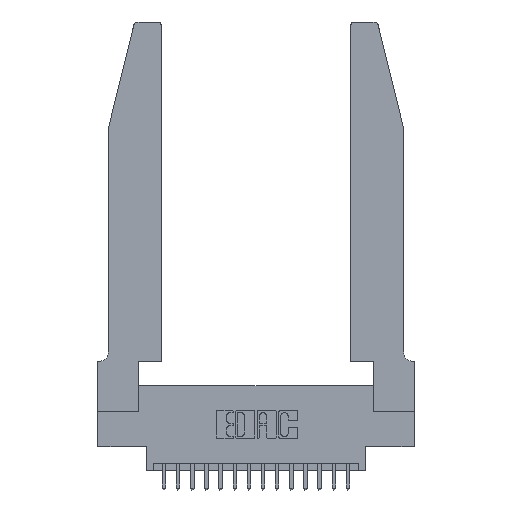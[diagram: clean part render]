
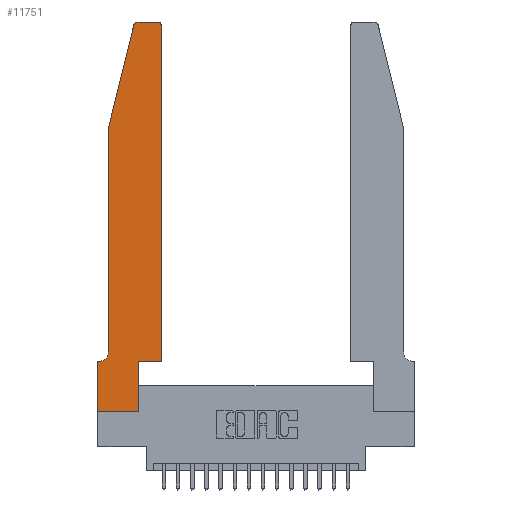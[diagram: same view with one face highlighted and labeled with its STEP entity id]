
A CAD part, top view. The second image highlights one B-rep face of the part: STEP entity #11751.
In plain terms, the highlighted planar face has unit normal (0, 0, 1).
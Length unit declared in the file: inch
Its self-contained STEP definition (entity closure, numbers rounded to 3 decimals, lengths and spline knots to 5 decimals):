
#253 = EDGE_CURVE ( 'NONE', #4071, #18024, #14234, .T. ) ;
#289 = ORIENTED_EDGE ( 'NONE', *, *, #15749, .T. ) ;
#462 = LINE ( 'NONE', #18966, #4676 ) ;
#570 = DIRECTION ( 'NONE',  ( -1., 0., 0. ) ) ;
#686 = CARTESIAN_POINT ( 'NONE',  ( 0.4205, 2.72, 0.37 ) ) ;
#854 = DIRECTION ( 'NONE',  ( 0., 1., 0. ) ) ;
#1380 = VECTOR ( 'NONE', #854, 39.37008 ) ;
#1409 = VERTEX_POINT ( 'NONE', #7134 ) ;
#2099 = DIRECTION ( 'NONE',  ( 1., 0., 0. ) ) ;
#2106 = CARTESIAN_POINT ( 'NONE',  ( 0.4505, 2.72, 0.37 ) ) ;
#2364 = EDGE_CURVE ( 'NONE', #1409, #4262, #3921, .T. ) ;
#2713 = DIRECTION ( 'NONE',  ( 0., 0., 1. ) ) ;
#3007 = CARTESIAN_POINT ( 'NONE',  ( 0.0755, 0.42, 0.37 ) ) ;
#3080 = AXIS2_PLACEMENT_3D ( 'NONE', #18809, #3494, #2099 ) ;
#3386 = CARTESIAN_POINT ( 'NONE',  ( 0.4505, 0.35, 0.37 ) ) ;
#3494 = DIRECTION ( 'NONE',  ( 0., 0., 1. ) ) ;
#3921 = LINE ( 'NONE', #7067, #4864 ) ;
#4011 = LINE ( 'NONE', #5177, #17823 ) ;
#4071 = VERTEX_POINT ( 'NONE', #13182 ) ;
#4124 = VECTOR ( 'NONE', #8865, 39.37008 ) ;
#4262 = VERTEX_POINT ( 'NONE', #5559 ) ;
#4607 = CARTESIAN_POINT ( 'NONE',  ( 0.284, 2.75, 0.37 ) ) ;
#4676 = VECTOR ( 'NONE', #14594, 39.37008 ) ;
#4864 = VECTOR ( 'NONE', #7128, 39.37008 ) ;
#5177 = CARTESIAN_POINT ( 'NONE',  ( 0.0755, 2., 0.37 ) ) ;
#5319 = DIRECTION ( 'NONE',  ( -1., 0., 0. ) ) ;
#5559 = CARTESIAN_POINT ( 'NONE',  ( 0.2865, 0.35, 0.37 ) ) ;
#5970 = VERTEX_POINT ( 'NONE', #3386 ) ;
#6296 = AXIS2_PLACEMENT_3D ( 'NONE', #9546, #15736, #570 ) ;
#6404 = VERTEX_POINT ( 'NONE', #4607 ) ;
#6453 = LINE ( 'NONE', #15044, #16662 ) ;
#6507 = ORIENTED_EDGE ( 'NONE', *, *, #19569, .T. ) ;
#7016 = LINE ( 'NONE', #10164, #4124 ) ;
#7067 = CARTESIAN_POINT ( 'NONE',  ( 0.2865, 0.35, 0.37 ) ) ;
#7128 = DIRECTION ( 'NONE',  ( 0., 1., 0. ) ) ;
#7134 = CARTESIAN_POINT ( 'NONE',  ( 0.2865, 0., 0.37 ) ) ;
#7719 = CARTESIAN_POINT ( 'NONE',  ( 0.4205, 2.75, 0.37 ) ) ;
#7859 = CIRCLE ( 'NONE', #10123, 0.03 ) ;
#8383 = ORIENTED_EDGE ( 'NONE', *, *, #15446, .T. ) ;
#8570 = ORIENTED_EDGE ( 'NONE', *, *, #15423, .T. ) ;
#8583 = VERTEX_POINT ( 'NONE', #2106 ) ;
#8700 = AXIS2_PLACEMENT_3D ( 'NONE', #686, #12571, #12638 ) ;
#8865 = DIRECTION ( 'NONE',  ( 1., 0., 0. ) ) ;
#9129 = CIRCLE ( 'NONE', #8700, 0.03 ) ;
#9407 = VERTEX_POINT ( 'NONE', #9571 ) ;
#9546 = CARTESIAN_POINT ( 'NONE',  ( 0.0055, 0.42, 0.37 ) ) ;
#9571 = CARTESIAN_POINT ( 'NONE',  ( 0., 0., 0.37 ) ) ;
#9643 = CARTESIAN_POINT ( 'NONE',  ( 0.4505, 0.35, 0.37 ) ) ;
#9687 = EDGE_CURVE ( 'NONE', #6404, #13571, #7859, .T. ) ;
#9867 = ORIENTED_EDGE ( 'NONE', *, *, #14270, .T. ) ;
#10023 = ORIENTED_EDGE ( 'NONE', *, *, #9687, .T. ) ;
#10123 = AXIS2_PLACEMENT_3D ( 'NONE', #19251, #2713, #11781 ) ;
#10164 = CARTESIAN_POINT ( 'NONE',  ( 0., 0., 0.37 ) ) ;
#10514 = VERTEX_POINT ( 'NONE', #7719 ) ;
#10768 = VERTEX_POINT ( 'NONE', #3007 ) ;
#10984 = ORIENTED_EDGE ( 'NONE', *, *, #15340, .T. ) ;
#11023 = LINE ( 'NONE', #11282, #14147 ) ;
#11236 = EDGE_CURVE ( 'NONE', #10514, #6404, #462, .T. ) ;
#11282 = CARTESIAN_POINT ( 'NONE',  ( 0.0755, 2., 0.37 ) ) ;
#11750 = LINE ( 'NONE', #9643, #1380 ) ;
#11751 = ADVANCED_FACE ( 'NONE', ( #15880 ), #17257, .T. ) ;
#11781 = DIRECTION ( 'NONE',  ( 1., 0., 0. ) ) ;
#12402 = CIRCLE ( 'NONE', #6296, 0.07 ) ;
#12571 = DIRECTION ( 'NONE',  ( 0., 0., 1. ) ) ;
#12574 = ORIENTED_EDGE ( 'NONE', *, *, #18176, .T. ) ;
#12638 = DIRECTION ( 'NONE',  ( 1., 0., 0. ) ) ;
#13182 = CARTESIAN_POINT ( 'NONE',  ( 0.0055, 0.35, 0.37 ) ) ;
#13462 = CARTESIAN_POINT ( 'NONE',  ( 0.0755, 2., 0.37 ) ) ;
#13503 = EDGE_LOOP ( 'NONE', ( #19459, #10023, #9867, #6507, #8383, #15883, #8570, #289, #18403, #12574, #14313, #10984 ) ) ;
#13571 = VERTEX_POINT ( 'NONE', #18210 ) ;
#13632 = DIRECTION ( 'NONE',  ( 1., 0., 0. ) ) ;
#13658 = EDGE_CURVE ( 'NONE', #5970, #8583, #11750, .T. ) ;
#14147 = VECTOR ( 'NONE', #17528, 39.37008 ) ;
#14234 = LINE ( 'NONE', #18967, #15181 ) ;
#14270 = EDGE_CURVE ( 'NONE', #13571, #16366, #11023, .T. ) ;
#14313 = ORIENTED_EDGE ( 'NONE', *, *, #13658, .T. ) ;
#14594 = DIRECTION ( 'NONE',  ( -1., 0., 0. ) ) ;
#15044 = CARTESIAN_POINT ( 'NONE',  ( 0.4505, 0.35, 0.37 ) ) ;
#15181 = VECTOR ( 'NONE', #5319, 39.37008 ) ;
#15340 = EDGE_CURVE ( 'NONE', #8583, #10514, #9129, .T. ) ;
#15423 = EDGE_CURVE ( 'NONE', #18024, #9407, #16984, .T. ) ;
#15446 = EDGE_CURVE ( 'NONE', #10768, #4071, #12402, .T. ) ;
#15736 = DIRECTION ( 'NONE',  ( 0., 0., -1. ) ) ;
#15749 = EDGE_CURVE ( 'NONE', #9407, #1409, #7016, .T. ) ;
#15880 = FACE_OUTER_BOUND ( 'NONE', #13503, .T. ) ;
#15883 = ORIENTED_EDGE ( 'NONE', *, *, #253, .T. ) ;
#15952 = DIRECTION ( 'NONE',  ( 0., -1., 0. ) ) ;
#16268 = CARTESIAN_POINT ( 'NONE',  ( 0., 0.35, 0.37 ) ) ;
#16366 = VERTEX_POINT ( 'NONE', #13462 ) ;
#16662 = VECTOR ( 'NONE', #13632, 39.37008 ) ;
#16984 = LINE ( 'NONE', #18843, #17731 ) ;
#17257 = PLANE ( 'NONE',  #3080 ) ;
#17528 = DIRECTION ( 'NONE',  ( -0.239, -0.971, 0. ) ) ;
#17731 = VECTOR ( 'NONE', #18697, 39.37008 ) ;
#17823 = VECTOR ( 'NONE', #15952, 39.37008 ) ;
#18024 = VERTEX_POINT ( 'NONE', #16268 ) ;
#18176 = EDGE_CURVE ( 'NONE', #4262, #5970, #6453, .T. ) ;
#18210 = CARTESIAN_POINT ( 'NONE',  ( 0.25487, 2.72718, 0.37 ) ) ;
#18403 = ORIENTED_EDGE ( 'NONE', *, *, #2364, .T. ) ;
#18697 = DIRECTION ( 'NONE',  ( 0., -1., 0. ) ) ;
#18809 = CARTESIAN_POINT ( 'NONE',  ( 0., 0.35, 0.37 ) ) ;
#18843 = CARTESIAN_POINT ( 'NONE',  ( 0., 0., 0.37 ) ) ;
#18966 = CARTESIAN_POINT ( 'NONE',  ( 0.2605, 2.75, 0.37 ) ) ;
#18967 = CARTESIAN_POINT ( 'NONE',  ( 0.0755, 0.35, 0.37 ) ) ;
#19251 = CARTESIAN_POINT ( 'NONE',  ( 0.284, 2.72, 0.37 ) ) ;
#19459 = ORIENTED_EDGE ( 'NONE', *, *, #11236, .T. ) ;
#19569 = EDGE_CURVE ( 'NONE', #16366, #10768, #4011, .T. ) ;
